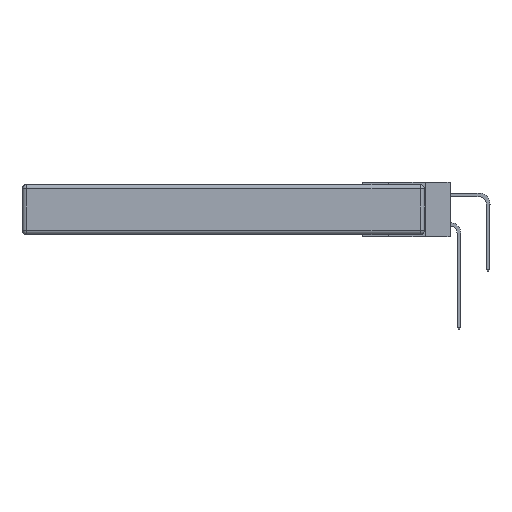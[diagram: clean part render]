
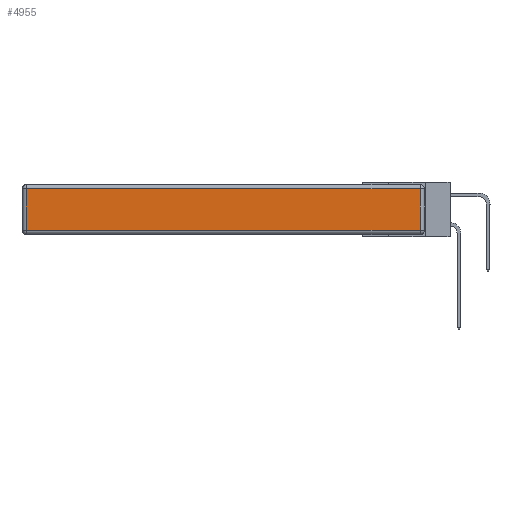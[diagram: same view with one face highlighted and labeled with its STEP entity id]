
A CAD part, left-side view. The second image highlights one B-rep face of the part: STEP entity #4955.
In plain terms, the highlighted planar face has unit normal (-1, 0, 0).
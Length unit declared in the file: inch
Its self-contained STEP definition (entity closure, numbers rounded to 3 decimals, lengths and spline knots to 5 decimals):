
#766 = DIRECTION ( 'NONE',  ( 0., 0., -1. ) ) ;
#2281 = VECTOR ( 'NONE', #36204, 39.37008 ) ;
#3569 = CARTESIAN_POINT ( 'NONE',  ( 0., 2.72, -0.343 ) ) ;
#4955 = ADVANCED_FACE ( 'NONE', ( #36890 ), #28817, .T. ) ;
#6829 = ORIENTED_EDGE ( 'NONE', *, *, #22815, .T. ) ;
#7251 = ORIENTED_EDGE ( 'NONE', *, *, #30069, .T. ) ;
#8357 = VECTOR ( 'NONE', #22698, 39.37008 ) ;
#8485 = CARTESIAN_POINT ( 'NONE',  ( 0., 0., -0.313 ) ) ;
#8986 = LINE ( 'NONE', #8485, #19050 ) ;
#9217 = VERTEX_POINT ( 'NONE', #18908 ) ;
#9270 = LINE ( 'NONE', #3569, #9747 ) ;
#9747 = VECTOR ( 'NONE', #766, 39.37008 ) ;
#10322 = ORIENTED_EDGE ( 'NONE', *, *, #33391, .T. ) ;
#10359 = CARTESIAN_POINT ( 'NONE',  ( 0., 2.72, -0.313 ) ) ;
#10978 = LINE ( 'NONE', #14247, #2281 ) ;
#11039 = DIRECTION ( 'NONE',  ( -1., 0., 0. ) ) ;
#11813 = EDGE_CURVE ( 'NONE', #9217, #27274, #10978, .T. ) ;
#13826 = VERTEX_POINT ( 'NONE', #10359 ) ;
#14116 = CARTESIAN_POINT ( 'NONE',  ( 0., 0.03, -0.343 ) ) ;
#14247 = CARTESIAN_POINT ( 'NONE',  ( 0., 2.75, -0.03 ) ) ;
#17025 = VERTEX_POINT ( 'NONE', #19785 ) ;
#18908 = CARTESIAN_POINT ( 'NONE',  ( 0., 0.03, -0.03 ) ) ;
#19050 = VECTOR ( 'NONE', #26901, 39.37008 ) ;
#19785 = CARTESIAN_POINT ( 'NONE',  ( 0., 0.03, -0.313 ) ) ;
#21951 = AXIS2_PLACEMENT_3D ( 'NONE', #26114, #11039, #22831 ) ;
#22698 = DIRECTION ( 'NONE',  ( 0., 0., 1. ) ) ;
#22815 = EDGE_CURVE ( 'NONE', #17025, #9217, #35367, .T. ) ;
#22831 = DIRECTION ( 'NONE',  ( 0., 0., 1. ) ) ;
#26114 = CARTESIAN_POINT ( 'NONE',  ( 0., 0., -0.343 ) ) ;
#26901 = DIRECTION ( 'NONE',  ( 0., -1., 0. ) ) ;
#27274 = VERTEX_POINT ( 'NONE', #30350 ) ;
#28817 = PLANE ( 'NONE',  #21951 ) ;
#30069 = EDGE_CURVE ( 'NONE', #13826, #17025, #8986, .T. ) ;
#30350 = CARTESIAN_POINT ( 'NONE',  ( 0., 2.72, -0.03 ) ) ;
#32802 = EDGE_LOOP ( 'NONE', ( #7251, #6829, #35262, #10322 ) ) ;
#33391 = EDGE_CURVE ( 'NONE', #27274, #13826, #9270, .T. ) ;
#35262 = ORIENTED_EDGE ( 'NONE', *, *, #11813, .T. ) ;
#35367 = LINE ( 'NONE', #14116, #8357 ) ;
#36204 = DIRECTION ( 'NONE',  ( 0., 1., 0. ) ) ;
#36890 = FACE_OUTER_BOUND ( 'NONE', #32802, .T. ) ;
